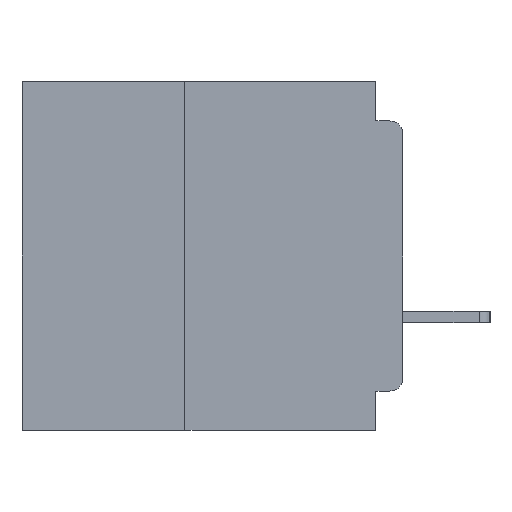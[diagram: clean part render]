
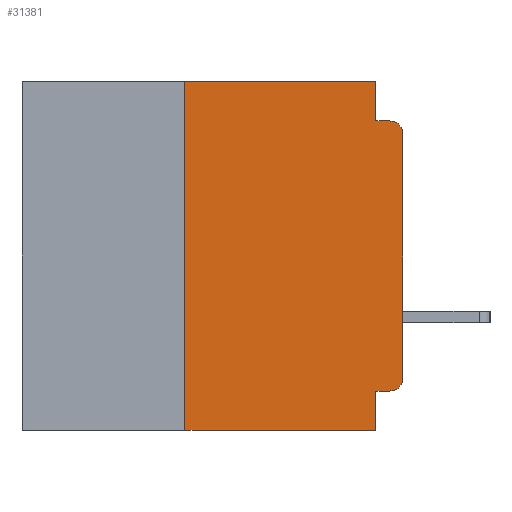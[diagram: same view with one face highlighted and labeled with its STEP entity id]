
A CAD part, left-side view. The second image highlights one B-rep face of the part: STEP entity #31381.
In plain terms, the highlighted planar face has unit normal (-1, 0, 0).
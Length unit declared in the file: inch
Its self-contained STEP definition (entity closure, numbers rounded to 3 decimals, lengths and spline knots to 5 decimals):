
#1263 = LINE ( 'NONE', #28923, #47017 ) ;
#1517 = CARTESIAN_POINT ( 'NONE',  ( 0., 0.031, 0. ) ) ;
#1659 = DIRECTION ( 'NONE',  ( 0., 0., -1. ) ) ;
#1688 = CARTESIAN_POINT ( 'NONE',  ( 0., 0.031, -0.4 ) ) ;
#1839 = FACE_OUTER_BOUND ( 'NONE', #36373, .T. ) ;
#1915 = LINE ( 'NONE', #15009, #30096 ) ;
#2233 = CARTESIAN_POINT ( 'NONE',  ( 0., 0.015, -0.06 ) ) ;
#3528 = CARTESIAN_POINT ( 'NONE',  ( 0., 0.031, -0.045 ) ) ;
#5876 = DIRECTION ( 'NONE',  ( 0., 1., 0. ) ) ;
#6310 = DIRECTION ( 'NONE',  ( 0., 0., -1. ) ) ;
#6505 = EDGE_CURVE ( 'NONE', #17475, #44435, #49533, .T. ) ;
#6853 = CIRCLE ( 'NONE', #39851, 0.015 ) ;
#7529 = VECTOR ( 'NONE', #50440, 39.37008 ) ;
#7656 = ORIENTED_EDGE ( 'NONE', *, *, #6505, .T. ) ;
#7881 = VECTOR ( 'NONE', #26371, 39.37008 ) ;
#8198 = AXIS2_PLACEMENT_3D ( 'NONE', #38653, #14712, #42716 ) ;
#8310 = CARTESIAN_POINT ( 'NONE',  ( 0., 0.015, -0.045 ) ) ;
#10199 = VERTEX_POINT ( 'NONE', #35425 ) ;
#13218 = ORIENTED_EDGE ( 'NONE', *, *, #18379, .T. ) ;
#14235 = EDGE_CURVE ( 'NONE', #17518, #24885, #51359, .T. ) ;
#14712 = DIRECTION ( 'NONE',  ( -1., 0., 0. ) ) ;
#15009 = CARTESIAN_POINT ( 'NONE',  ( 0., 0.031, -0.4 ) ) ;
#16047 = LINE ( 'NONE', #20056, #25369 ) ;
#16574 = EDGE_CURVE ( 'NONE', #32808, #37859, #6853, .T. ) ;
#16957 = CARTESIAN_POINT ( 'NONE',  ( 0., 0.437, 0. ) ) ;
#17475 = VERTEX_POINT ( 'NONE', #34256 ) ;
#17518 = VERTEX_POINT ( 'NONE', #38303 ) ;
#18379 = EDGE_CURVE ( 'NONE', #17518, #36807, #16047, .T. ) ;
#18731 = ORIENTED_EDGE ( 'NONE', *, *, #32373, .T. ) ;
#19368 = EDGE_CURVE ( 'NONE', #39995, #37859, #19768, .T. ) ;
#19768 = LINE ( 'NONE', #50237, #7881 ) ;
#19885 = VECTOR ( 'NONE', #5876, 39.37008 ) ;
#20056 = CARTESIAN_POINT ( 'NONE',  ( 0., 0.437, -0.4 ) ) ;
#20151 = CARTESIAN_POINT ( 'NONE',  ( 0., 0., 0. ) ) ;
#23549 = EDGE_CURVE ( 'NONE', #17475, #10199, #51848, .T. ) ;
#24022 = DIRECTION ( 'NONE',  ( 0., -1., 0. ) ) ;
#24111 = DIRECTION ( 'NONE',  ( 0., 0., 1. ) ) ;
#24346 = ORIENTED_EDGE ( 'NONE', *, *, #19368, .F. ) ;
#24395 = ORIENTED_EDGE ( 'NONE', *, *, #14235, .F. ) ;
#24885 = VERTEX_POINT ( 'NONE', #43033 ) ;
#25369 = VECTOR ( 'NONE', #24022, 39.37008 ) ;
#25626 = DIRECTION ( 'NONE',  ( 1., 0., 0. ) ) ;
#26371 = DIRECTION ( 'NONE',  ( 0., -1., 0. ) ) ;
#28923 = CARTESIAN_POINT ( 'NONE',  ( 0., 0.031, 0. ) ) ;
#28957 = DIRECTION ( 'NONE',  ( 0., -1., 0. ) ) ;
#29377 = ORIENTED_EDGE ( 'NONE', *, *, #39595, .F. ) ;
#29812 = CARTESIAN_POINT ( 'NONE',  ( 0., 0., -0.355 ) ) ;
#30096 = VECTOR ( 'NONE', #47054, 39.37008 ) ;
#30246 = DIRECTION ( 'NONE',  ( -1., 0., 0. ) ) ;
#30292 = CARTESIAN_POINT ( 'NONE',  ( 0., 0.25, -0.4 ) ) ;
#30927 = CARTESIAN_POINT ( 'NONE',  ( 0., 0., -0.06 ) ) ;
#31381 = ADVANCED_FACE ( 'NONE', ( #1839 ), #41598, .F. ) ;
#32373 = EDGE_CURVE ( 'NONE', #44435, #32808, #35515, .T. ) ;
#32386 = VECTOR ( 'NONE', #28957, 39.37008 ) ;
#32808 = VERTEX_POINT ( 'NONE', #30927 ) ;
#32956 = DIRECTION ( 'NONE',  ( 0., 0., -1. ) ) ;
#33867 = VERTEX_POINT ( 'NONE', #1517 ) ;
#34238 = VECTOR ( 'NONE', #24111, 39.37008 ) ;
#34256 = CARTESIAN_POINT ( 'NONE',  ( 0., 0.015, -0.355 ) ) ;
#34400 = ORIENTED_EDGE ( 'NONE', *, *, #35589, .F. ) ;
#35425 = CARTESIAN_POINT ( 'NONE',  ( 0., 0.031, -0.355 ) ) ;
#35515 = LINE ( 'NONE', #20151, #34238 ) ;
#35589 = EDGE_CURVE ( 'NONE', #24885, #33867, #43075, .T. ) ;
#36373 = EDGE_LOOP ( 'NONE', ( #18731, #43198, #24346, #29377, #34400, #24395, #13218, #36963, #43966, #7656 ) ) ;
#36807 = VERTEX_POINT ( 'NONE', #1688 ) ;
#36963 = ORIENTED_EDGE ( 'NONE', *, *, #39293, .F. ) ;
#37532 = CARTESIAN_POINT ( 'NONE',  ( 0., 0.437, 0. ) ) ;
#37859 = VERTEX_POINT ( 'NONE', #8310 ) ;
#38303 = CARTESIAN_POINT ( 'NONE',  ( 0., 0.25, -0.4 ) ) ;
#38653 = CARTESIAN_POINT ( 'NONE',  ( 0., 0.015, -0.34 ) ) ;
#39293 = EDGE_CURVE ( 'NONE', #10199, #36807, #1915, .T. ) ;
#39595 = EDGE_CURVE ( 'NONE', #33867, #39995, #1263, .T. ) ;
#39696 = AXIS2_PLACEMENT_3D ( 'NONE', #37532, #25626, #1659 ) ;
#39851 = AXIS2_PLACEMENT_3D ( 'NONE', #2233, #30246, #6310 ) ;
#39995 = VERTEX_POINT ( 'NONE', #3528 ) ;
#41598 = PLANE ( 'NONE',  #39696 ) ;
#42716 = DIRECTION ( 'NONE',  ( 0., 0., -1. ) ) ;
#43033 = CARTESIAN_POINT ( 'NONE',  ( 0., 0.25, 0. ) ) ;
#43075 = LINE ( 'NONE', #16957, #32386 ) ;
#43198 = ORIENTED_EDGE ( 'NONE', *, *, #16574, .T. ) ;
#43966 = ORIENTED_EDGE ( 'NONE', *, *, #23549, .F. ) ;
#44174 = CARTESIAN_POINT ( 'NONE',  ( 0., 0., -0.34 ) ) ;
#44435 = VERTEX_POINT ( 'NONE', #44174 ) ;
#47017 = VECTOR ( 'NONE', #32956, 39.37008 ) ;
#47054 = DIRECTION ( 'NONE',  ( 0., 0., -1. ) ) ;
#49533 = CIRCLE ( 'NONE', #8198, 0.015 ) ;
#50237 = CARTESIAN_POINT ( 'NONE',  ( 0., 0., -0.045 ) ) ;
#50440 = DIRECTION ( 'NONE',  ( 0., 0., 1. ) ) ;
#51359 = LINE ( 'NONE', #30292, #7529 ) ;
#51848 = LINE ( 'NONE', #29812, #19885 ) ;
